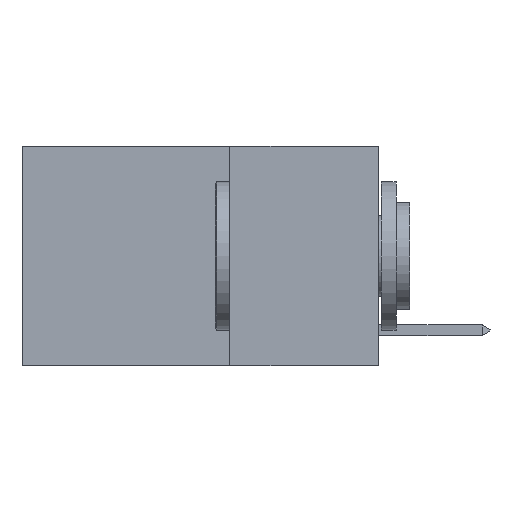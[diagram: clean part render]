
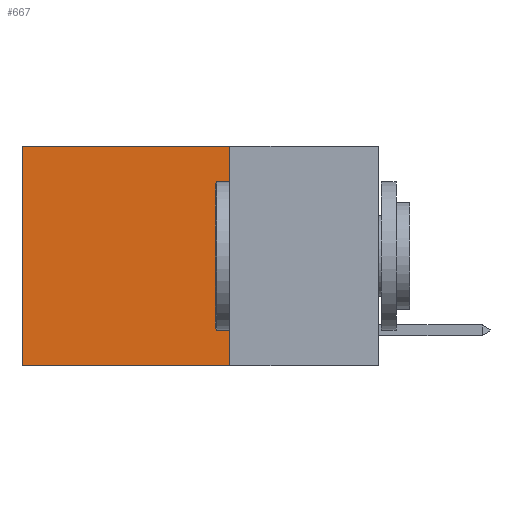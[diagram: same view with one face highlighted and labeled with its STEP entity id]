
A CAD part, left-side view. The second image highlights one B-rep face of the part: STEP entity #667.
In plain terms, the highlighted planar face has unit normal (-1, 0, 0).
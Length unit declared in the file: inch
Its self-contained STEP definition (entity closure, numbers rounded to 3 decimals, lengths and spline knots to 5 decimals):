
#223 = CARTESIAN_POINT ( 'NONE',  ( 0.2625, 0.6, 0. ) ) ;
#667 = ADVANCED_FACE ( 'NONE', ( #6073 ), #3967, .F. ) ;
#688 = CARTESIAN_POINT ( 'NONE',  ( 0.2625, 0.25, 0. ) ) ;
#1055 = EDGE_CURVE ( 'NONE', #11995, #2269, #12581, .T. ) ;
#1194 = EDGE_LOOP ( 'NONE', ( #11464, #6094, #8569, #6774 ) ) ;
#1775 = DIRECTION ( 'NONE',  ( 1., 0., 0. ) ) ;
#2055 = LINE ( 'NONE', #10802, #9956 ) ;
#2269 = VERTEX_POINT ( 'NONE', #3690 ) ;
#2588 = AXIS2_PLACEMENT_3D ( 'NONE', #688, #1775, #12540 ) ;
#2715 = LINE ( 'NONE', #7133, #11531 ) ;
#2894 = CARTESIAN_POINT ( 'NONE',  ( 0.2625, 0.6, 0. ) ) ;
#3690 = CARTESIAN_POINT ( 'NONE',  ( 0.2625, 0.6, -0.37 ) ) ;
#3967 = PLANE ( 'NONE',  #2588 ) ;
#5763 = VERTEX_POINT ( 'NONE', #7709 ) ;
#6073 = FACE_OUTER_BOUND ( 'NONE', #1194, .T. ) ;
#6094 = ORIENTED_EDGE ( 'NONE', *, *, #11942, .F. ) ;
#6774 = ORIENTED_EDGE ( 'NONE', *, *, #10406, .T. ) ;
#6875 = LINE ( 'NONE', #8146, #13567 ) ;
#6925 = EDGE_CURVE ( 'NONE', #5763, #8712, #6875, .T. ) ;
#6984 = VECTOR ( 'NONE', #7105, 39.37008 ) ;
#7105 = DIRECTION ( 'NONE',  ( 0., 0., -1. ) ) ;
#7133 = CARTESIAN_POINT ( 'NONE',  ( 0.2625, 0.25, 0. ) ) ;
#7709 = CARTESIAN_POINT ( 'NONE',  ( 0.2625, 0.25, 0. ) ) ;
#8146 = CARTESIAN_POINT ( 'NONE',  ( 0.2625, 0.25, 0. ) ) ;
#8569 = ORIENTED_EDGE ( 'NONE', *, *, #6925, .F. ) ;
#8676 = DIRECTION ( 'NONE',  ( 0., 1., 0. ) ) ;
#8712 = VERTEX_POINT ( 'NONE', #13493 ) ;
#9956 = VECTOR ( 'NONE', #8676, 39.37008 ) ;
#10406 = EDGE_CURVE ( 'NONE', #5763, #11995, #2715, .T. ) ;
#10802 = CARTESIAN_POINT ( 'NONE',  ( 0.2625, 0.25, -0.37 ) ) ;
#11461 = DIRECTION ( 'NONE',  ( 0., 1., 0. ) ) ;
#11464 = ORIENTED_EDGE ( 'NONE', *, *, #1055, .T. ) ;
#11531 = VECTOR ( 'NONE', #11461, 39.37008 ) ;
#11942 = EDGE_CURVE ( 'NONE', #8712, #2269, #2055, .T. ) ;
#11995 = VERTEX_POINT ( 'NONE', #223 ) ;
#12499 = DIRECTION ( 'NONE',  ( 0., 0., -1. ) ) ;
#12540 = DIRECTION ( 'NONE',  ( 0., 0., -1. ) ) ;
#12581 = LINE ( 'NONE', #2894, #6984 ) ;
#13493 = CARTESIAN_POINT ( 'NONE',  ( 0.2625, 0.25, -0.37 ) ) ;
#13567 = VECTOR ( 'NONE', #12499, 39.37008 ) ;
